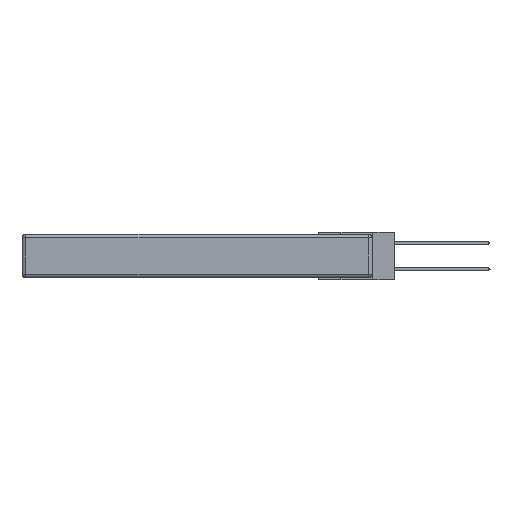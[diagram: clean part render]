
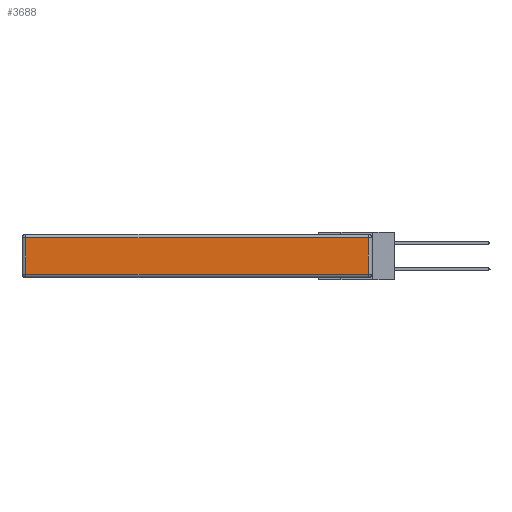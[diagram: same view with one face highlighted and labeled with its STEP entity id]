
A CAD part, left-side view. The second image highlights one B-rep face of the part: STEP entity #3688.
In plain terms, the highlighted planar face has unit normal (-1, 0, 0).
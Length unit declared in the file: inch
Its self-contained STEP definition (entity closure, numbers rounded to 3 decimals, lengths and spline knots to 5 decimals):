
#338 = LINE ( 'NONE', #15315, #1737 ) ;
#520 = CARTESIAN_POINT ( 'NONE',  ( 0., 0.03, -0.343 ) ) ;
#777 = EDGE_CURVE ( 'NONE', #16131, #12770, #15732, .T. ) ;
#857 = FACE_OUTER_BOUND ( 'NONE', #4018, .T. ) ;
#1640 = ORIENTED_EDGE ( 'NONE', *, *, #6082, .T. ) ;
#1737 = VECTOR ( 'NONE', #3005, 39.37008 ) ;
#2456 = EDGE_CURVE ( 'NONE', #12770, #6948, #3932, .T. ) ;
#2641 = DIRECTION ( 'NONE',  ( -1., 0., 0. ) ) ;
#2838 = CARTESIAN_POINT ( 'NONE',  ( 0., 2.72, -0.313 ) ) ;
#3005 = DIRECTION ( 'NONE',  ( 0., 1., 0. ) ) ;
#3688 = ADVANCED_FACE ( 'NONE', ( #857 ), #5748, .T. ) ;
#3932 = LINE ( 'NONE', #14062, #14282 ) ;
#4018 = EDGE_LOOP ( 'NONE', ( #10142, #1640, #20663, #15823 ) ) ;
#4051 = DIRECTION ( 'NONE',  ( 0., 0., 1. ) ) ;
#5748 = PLANE ( 'NONE',  #9646 ) ;
#5844 = CARTESIAN_POINT ( 'NONE',  ( 0., 0.03, -0.03 ) ) ;
#6082 = EDGE_CURVE ( 'NONE', #6948, #10593, #20539, .T. ) ;
#6948 = VERTEX_POINT ( 'NONE', #8862 ) ;
#8862 = CARTESIAN_POINT ( 'NONE',  ( 0., 0.03, -0.313 ) ) ;
#8963 = CARTESIAN_POINT ( 'NONE',  ( 0., 2.72, -0.343 ) ) ;
#9646 = AXIS2_PLACEMENT_3D ( 'NONE', #11571, #2641, #15100 ) ;
#10142 = ORIENTED_EDGE ( 'NONE', *, *, #2456, .T. ) ;
#10593 = VERTEX_POINT ( 'NONE', #5844 ) ;
#11571 = CARTESIAN_POINT ( 'NONE',  ( 0., 0., -0.343 ) ) ;
#12770 = VERTEX_POINT ( 'NONE', #2838 ) ;
#13445 = CARTESIAN_POINT ( 'NONE',  ( 0., 2.72, -0.03 ) ) ;
#14062 = CARTESIAN_POINT ( 'NONE',  ( 0., 0., -0.313 ) ) ;
#14282 = VECTOR ( 'NONE', #19450, 39.37008 ) ;
#15100 = DIRECTION ( 'NONE',  ( 0., 0., 1. ) ) ;
#15189 = VECTOR ( 'NONE', #16090, 39.37008 ) ;
#15315 = CARTESIAN_POINT ( 'NONE',  ( 0., 2.75, -0.03 ) ) ;
#15732 = LINE ( 'NONE', #8963, #15189 ) ;
#15823 = ORIENTED_EDGE ( 'NONE', *, *, #777, .T. ) ;
#15972 = EDGE_CURVE ( 'NONE', #10593, #16131, #338, .T. ) ;
#16090 = DIRECTION ( 'NONE',  ( 0., 0., -1. ) ) ;
#16131 = VERTEX_POINT ( 'NONE', #13445 ) ;
#17993 = VECTOR ( 'NONE', #4051, 39.37008 ) ;
#19450 = DIRECTION ( 'NONE',  ( 0., -1., 0. ) ) ;
#20539 = LINE ( 'NONE', #520, #17993 ) ;
#20663 = ORIENTED_EDGE ( 'NONE', *, *, #15972, .T. ) ;
